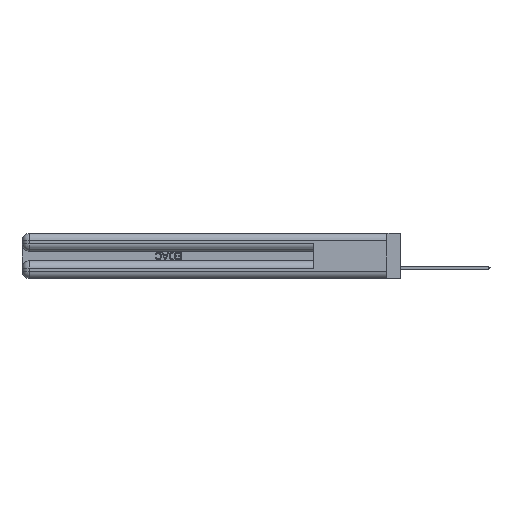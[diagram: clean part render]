
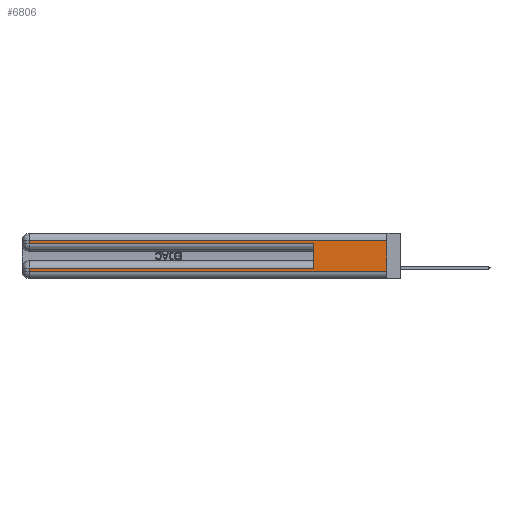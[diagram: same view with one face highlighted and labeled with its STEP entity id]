
A CAD part, left-side view. The second image highlights one B-rep face of the part: STEP entity #6806.
In plain terms, the highlighted planar face has unit normal (-1, 0, 0).
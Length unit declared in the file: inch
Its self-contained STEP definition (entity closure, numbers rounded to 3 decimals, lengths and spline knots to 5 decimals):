
#905 = LINE ( 'NONE', #39451, #38998 ) ;
#2279 = CARTESIAN_POINT ( 'NONE',  ( 0., 0.6, 0.085 ) ) ;
#2348 = CARTESIAN_POINT ( 'NONE',  ( 0., 0.6, 0.145 ) ) ;
#3225 = VECTOR ( 'NONE', #45454, 39.37008 ) ;
#4028 = LINE ( 'NONE', #31867, #38259 ) ;
#5661 = EDGE_CURVE ( 'NONE', #17939, #24117, #13858, .T. ) ;
#5982 = ORIENTED_EDGE ( 'NONE', *, *, #26954, .T. ) ;
#6309 = VERTEX_POINT ( 'NONE', #2279 ) ;
#6496 = CARTESIAN_POINT ( 'NONE',  ( 0., 0., 0.06 ) ) ;
#6654 = DIRECTION ( 'NONE',  ( 1., 0., 0. ) ) ;
#6806 = ADVANCED_FACE ( 'NONE', ( #33159 ), #44871, .F. ) ;
#7030 = DIRECTION ( 'NONE',  ( 0., -1., 0. ) ) ;
#8653 = CARTESIAN_POINT ( 'NONE',  ( 0., 2.94, 0.31 ) ) ;
#9474 = VECTOR ( 'NONE', #7030, 39.37008 ) ;
#9572 = CARTESIAN_POINT ( 'NONE',  ( 0., 2.94, 0.085 ) ) ;
#9594 = CARTESIAN_POINT ( 'NONE',  ( 0., 0., 0.37 ) ) ;
#9645 = EDGE_CURVE ( 'NONE', #6309, #32093, #34558, .T. ) ;
#10181 = DIRECTION ( 'NONE',  ( 0., 0., -1. ) ) ;
#10431 = VERTEX_POINT ( 'NONE', #9572 ) ;
#11941 = CARTESIAN_POINT ( 'NONE',  ( 0., 0.6, 0.285 ) ) ;
#12598 = ORIENTED_EDGE ( 'NONE', *, *, #40355, .T. ) ;
#13730 = CARTESIAN_POINT ( 'NONE',  ( 0., 0., 0.31 ) ) ;
#13858 = LINE ( 'NONE', #38960, #9474 ) ;
#14352 = DIRECTION ( 'NONE',  ( 0., 1., 0. ) ) ;
#14631 = CARTESIAN_POINT ( 'NONE',  ( 0., 2.94, 0.37 ) ) ;
#15073 = DIRECTION ( 'NONE',  ( 0., -1., 0. ) ) ;
#17939 = VERTEX_POINT ( 'NONE', #33428 ) ;
#19854 = VERTEX_POINT ( 'NONE', #36072 ) ;
#20524 = DIRECTION ( 'NONE',  ( 0., 0., -1. ) ) ;
#20805 = CARTESIAN_POINT ( 'NONE',  ( 0., 2.94, 0.37 ) ) ;
#20866 = ORIENTED_EDGE ( 'NONE', *, *, #39976, .T. ) ;
#21040 = VECTOR ( 'NONE', #43149, 39.37008 ) ;
#21163 = EDGE_CURVE ( 'NONE', #29916, #24117, #31518, .T. ) ;
#21916 = LINE ( 'NONE', #20805, #3225 ) ;
#22588 = VECTOR ( 'NONE', #10181, 39.37008 ) ;
#23114 = VERTEX_POINT ( 'NONE', #8653 ) ;
#24117 = VERTEX_POINT ( 'NONE', #6496 ) ;
#25422 = LINE ( 'NONE', #44407, #31554 ) ;
#26954 = EDGE_CURVE ( 'NONE', #6309, #10431, #4028, .T. ) ;
#27170 = CARTESIAN_POINT ( 'NONE',  ( 0., 0., 0.37 ) ) ;
#27402 = ORIENTED_EDGE ( 'NONE', *, *, #9645, .F. ) ;
#29048 = ORIENTED_EDGE ( 'NONE', *, *, #45009, .T. ) ;
#29916 = VERTEX_POINT ( 'NONE', #13730 ) ;
#31518 = LINE ( 'NONE', #9594, #22588 ) ;
#31554 = VECTOR ( 'NONE', #33867, 39.37008 ) ;
#31867 = CARTESIAN_POINT ( 'NONE',  ( 0., 0., 0.085 ) ) ;
#32093 = VERTEX_POINT ( 'NONE', #11941 ) ;
#33159 = FACE_OUTER_BOUND ( 'NONE', #37994, .T. ) ;
#33188 = ORIENTED_EDGE ( 'NONE', *, *, #5661, .T. ) ;
#33428 = CARTESIAN_POINT ( 'NONE',  ( 0., 2.94, 0.06 ) ) ;
#33867 = DIRECTION ( 'NONE',  ( 0., 1., 0. ) ) ;
#34558 = LINE ( 'NONE', #2348, #38367 ) ;
#35036 = EDGE_CURVE ( 'NONE', #19854, #32093, #905, .T. ) ;
#35826 = ORIENTED_EDGE ( 'NONE', *, *, #35036, .T. ) ;
#36072 = CARTESIAN_POINT ( 'NONE',  ( 0., 2.94, 0.285 ) ) ;
#36499 = AXIS2_PLACEMENT_3D ( 'NONE', #27170, #6654, #20524 ) ;
#37994 = EDGE_LOOP ( 'NONE', ( #44777, #12598, #20866, #35826, #27402, #5982, #29048, #33188 ) ) ;
#38259 = VECTOR ( 'NONE', #14352, 39.37008 ) ;
#38367 = VECTOR ( 'NONE', #45157, 39.37008 ) ;
#38960 = CARTESIAN_POINT ( 'NONE',  ( 0., 0., 0.06 ) ) ;
#38998 = VECTOR ( 'NONE', #15073, 39.37008 ) ;
#39451 = CARTESIAN_POINT ( 'NONE',  ( 0., 0., 0.285 ) ) ;
#39976 = EDGE_CURVE ( 'NONE', #23114, #19854, #42008, .T. ) ;
#40355 = EDGE_CURVE ( 'NONE', #29916, #23114, #25422, .T. ) ;
#42008 = LINE ( 'NONE', #14631, #21040 ) ;
#43149 = DIRECTION ( 'NONE',  ( 0., 0., -1. ) ) ;
#44407 = CARTESIAN_POINT ( 'NONE',  ( 0., 0., 0.31 ) ) ;
#44777 = ORIENTED_EDGE ( 'NONE', *, *, #21163, .F. ) ;
#44871 = PLANE ( 'NONE',  #36499 ) ;
#45009 = EDGE_CURVE ( 'NONE', #10431, #17939, #21916, .T. ) ;
#45157 = DIRECTION ( 'NONE',  ( 0., 0., 1. ) ) ;
#45454 = DIRECTION ( 'NONE',  ( 0., 0., -1. ) ) ;
